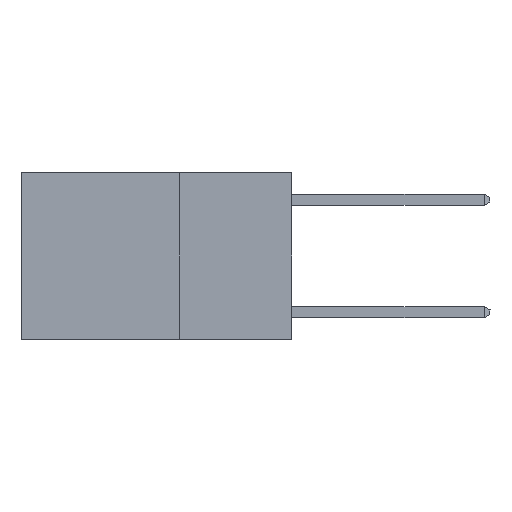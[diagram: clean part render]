
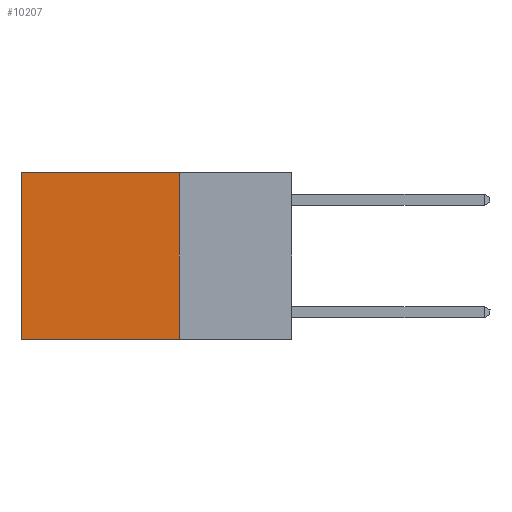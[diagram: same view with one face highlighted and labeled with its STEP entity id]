
A CAD part, left-side view. The second image highlights one B-rep face of the part: STEP entity #10207.
In plain terms, the highlighted planar face has unit normal (-1, 0, 0).
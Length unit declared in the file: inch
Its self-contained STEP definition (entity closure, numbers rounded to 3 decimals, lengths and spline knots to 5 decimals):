
#65 = VERTEX_POINT ( 'NONE', #6693 ) ;
#1078 = CARTESIAN_POINT ( 'NONE',  ( 0.2625, 0.25, -0.37 ) ) ;
#1388 = CARTESIAN_POINT ( 'NONE',  ( 0.2625, 0.25, 0. ) ) ;
#2962 = VECTOR ( 'NONE', #5235, 39.37008 ) ;
#3921 = VECTOR ( 'NONE', #15058, 39.37008 ) ;
#4201 = VERTEX_POINT ( 'NONE', #21037 ) ;
#4353 = CARTESIAN_POINT ( 'NONE',  ( 0.2625, 0.6, 0. ) ) ;
#4360 = ORIENTED_EDGE ( 'NONE', *, *, #14270, .T. ) ;
#4840 = VERTEX_POINT ( 'NONE', #19247 ) ;
#5235 = DIRECTION ( 'NONE',  ( 0., 0., -1. ) ) ;
#5354 = ORIENTED_EDGE ( 'NONE', *, *, #17584, .T. ) ;
#5671 = CARTESIAN_POINT ( 'NONE',  ( 0.2625, 0.25, -0.37 ) ) ;
#6693 = CARTESIAN_POINT ( 'NONE',  ( 0.2625, 0.25, 0. ) ) ;
#7250 = CARTESIAN_POINT ( 'NONE',  ( 0.2625, 0.25, 0. ) ) ;
#8487 = DIRECTION ( 'NONE',  ( 0., 1., 0. ) ) ;
#9078 = DIRECTION ( 'NONE',  ( 1., 0., 0. ) ) ;
#10124 = EDGE_CURVE ( 'NONE', #65, #15472, #17203, .T. ) ;
#10207 = ADVANCED_FACE ( 'NONE', ( #12618 ), #19479, .F. ) ;
#12618 = FACE_OUTER_BOUND ( 'NONE', #18939, .T. ) ;
#13442 = VECTOR ( 'NONE', #8487, 39.37008 ) ;
#13512 = LINE ( 'NONE', #4353, #3921 ) ;
#14168 = ORIENTED_EDGE ( 'NONE', *, *, #10124, .F. ) ;
#14270 = EDGE_CURVE ( 'NONE', #4201, #4840, #13512, .T. ) ;
#15058 = DIRECTION ( 'NONE',  ( 0., 0., -1. ) ) ;
#15472 = VERTEX_POINT ( 'NONE', #5671 ) ;
#15536 = EDGE_CURVE ( 'NONE', #15472, #4840, #18017, .T. ) ;
#16471 = ORIENTED_EDGE ( 'NONE', *, *, #15536, .F. ) ;
#17148 = AXIS2_PLACEMENT_3D ( 'NONE', #7250, #9078, #21157 ) ;
#17203 = LINE ( 'NONE', #20874, #2962 ) ;
#17415 = VECTOR ( 'NONE', #17519, 39.37008 ) ;
#17519 = DIRECTION ( 'NONE',  ( 0., 1., 0. ) ) ;
#17584 = EDGE_CURVE ( 'NONE', #65, #4201, #17941, .T. ) ;
#17941 = LINE ( 'NONE', #1388, #17415 ) ;
#18017 = LINE ( 'NONE', #1078, #13442 ) ;
#18939 = EDGE_LOOP ( 'NONE', ( #4360, #16471, #14168, #5354 ) ) ;
#19247 = CARTESIAN_POINT ( 'NONE',  ( 0.2625, 0.6, -0.37 ) ) ;
#19479 = PLANE ( 'NONE',  #17148 ) ;
#20874 = CARTESIAN_POINT ( 'NONE',  ( 0.2625, 0.25, 0. ) ) ;
#21037 = CARTESIAN_POINT ( 'NONE',  ( 0.2625, 0.6, 0. ) ) ;
#21157 = DIRECTION ( 'NONE',  ( 0., 0., -1. ) ) ;
